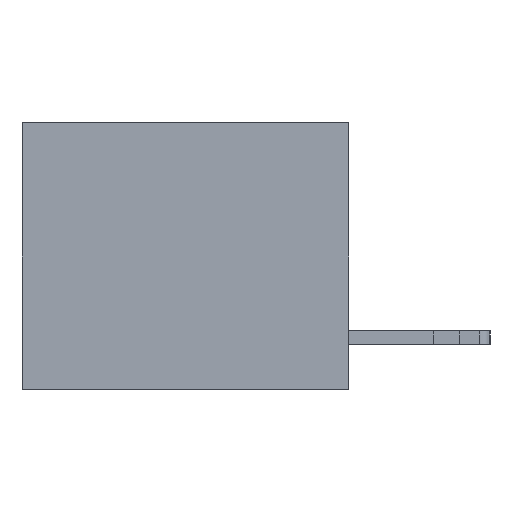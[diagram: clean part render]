
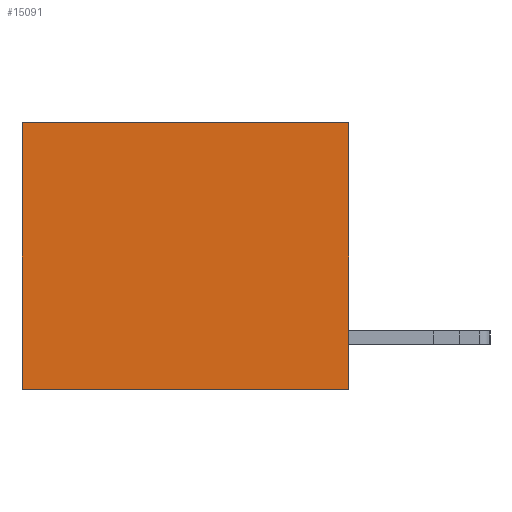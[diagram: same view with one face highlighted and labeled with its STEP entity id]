
A CAD part, left-side view. The second image highlights one B-rep face of the part: STEP entity #15091.
In plain terms, the highlighted planar face has unit normal (-1, 0, 0).
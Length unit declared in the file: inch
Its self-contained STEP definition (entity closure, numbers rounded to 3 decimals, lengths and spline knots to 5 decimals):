
#542 = VERTEX_POINT ( 'NONE', #28605 ) ;
#892 = ORIENTED_EDGE ( 'NONE', *, *, #26744, .F. ) ;
#1578 = VECTOR ( 'NONE', #28296, 39.37008 ) ;
#1686 = DIRECTION ( 'NONE',  ( 0., 0., -1. ) ) ;
#2036 = CARTESIAN_POINT ( 'NONE',  ( 0.3165, 0.6, 0. ) ) ;
#2409 = CARTESIAN_POINT ( 'NONE',  ( 0.3165, 0., -0.49 ) ) ;
#4370 = LINE ( 'NONE', #2409, #10250 ) ;
#6286 = VECTOR ( 'NONE', #11195, 39.37008 ) ;
#7001 = EDGE_CURVE ( 'NONE', #12534, #9957, #12209, .T. ) ;
#7036 = DIRECTION ( 'NONE',  ( 0., 0., -1. ) ) ;
#7148 = VERTEX_POINT ( 'NONE', #19747 ) ;
#7544 = ORIENTED_EDGE ( 'NONE', *, *, #20563, .F. ) ;
#8747 = CARTESIAN_POINT ( 'NONE',  ( 0.3165, 0.6, -0.49 ) ) ;
#9140 = ORIENTED_EDGE ( 'NONE', *, *, #23894, .T. ) ;
#9957 = VERTEX_POINT ( 'NONE', #22544 ) ;
#10250 = VECTOR ( 'NONE', #7036, 39.37008 ) ;
#11195 = DIRECTION ( 'NONE',  ( 0., 0., -1. ) ) ;
#11655 = CARTESIAN_POINT ( 'NONE',  ( 0.3165, 0., -0.49 ) ) ;
#11735 = FACE_OUTER_BOUND ( 'NONE', #23600, .T. ) ;
#12209 = LINE ( 'NONE', #8747, #6286 ) ;
#12451 = CARTESIAN_POINT ( 'NONE',  ( 0.3165, 0., -0.49 ) ) ;
#12534 = VERTEX_POINT ( 'NONE', #2036 ) ;
#12719 = PLANE ( 'NONE',  #24627 ) ;
#14683 = DIRECTION ( 'NONE',  ( 1., 0., 0. ) ) ;
#15091 = ADVANCED_FACE ( 'NONE', ( #11735 ), #12719, .F. ) ;
#17337 = CARTESIAN_POINT ( 'NONE',  ( 0.3165, 0., 0. ) ) ;
#19421 = LINE ( 'NONE', #11655, #21496 ) ;
#19747 = CARTESIAN_POINT ( 'NONE',  ( 0.3165, 0., 0. ) ) ;
#20563 = EDGE_CURVE ( 'NONE', #542, #9957, #19421, .T. ) ;
#21496 = VECTOR ( 'NONE', #22594, 39.37008 ) ;
#22544 = CARTESIAN_POINT ( 'NONE',  ( 0.3165, 0.6, -0.49 ) ) ;
#22594 = DIRECTION ( 'NONE',  ( 0., 1., 0. ) ) ;
#23600 = EDGE_LOOP ( 'NONE', ( #26905, #7544, #892, #9140 ) ) ;
#23894 = EDGE_CURVE ( 'NONE', #7148, #12534, #24151, .T. ) ;
#24151 = LINE ( 'NONE', #17337, #1578 ) ;
#24627 = AXIS2_PLACEMENT_3D ( 'NONE', #12451, #14683, #1686 ) ;
#26744 = EDGE_CURVE ( 'NONE', #7148, #542, #4370, .T. ) ;
#26905 = ORIENTED_EDGE ( 'NONE', *, *, #7001, .T. ) ;
#28296 = DIRECTION ( 'NONE',  ( 0., 1., 0. ) ) ;
#28605 = CARTESIAN_POINT ( 'NONE',  ( 0.3165, 0., -0.49 ) ) ;
